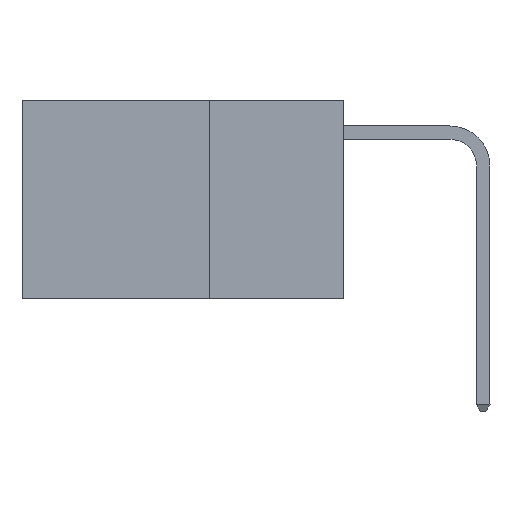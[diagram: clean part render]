
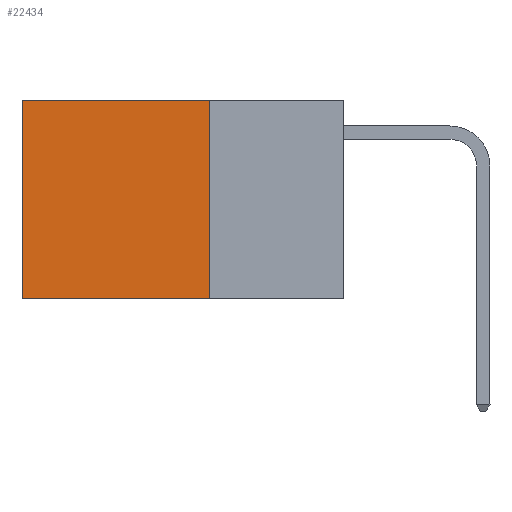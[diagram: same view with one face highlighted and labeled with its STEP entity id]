
A CAD part, left-side view. The second image highlights one B-rep face of the part: STEP entity #22434.
In plain terms, the highlighted planar face has unit normal (-1, 0, 0).
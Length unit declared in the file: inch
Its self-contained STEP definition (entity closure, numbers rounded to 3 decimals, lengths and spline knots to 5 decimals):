
#452 = VERTEX_POINT ( 'NONE', #15497 ) ;
#905 = DIRECTION ( 'NONE',  ( 0., 0., -1. ) ) ;
#1413 = ORIENTED_EDGE ( 'NONE', *, *, #18314, .T. ) ;
#1523 = ORIENTED_EDGE ( 'NONE', *, *, #17590, .F. ) ;
#2124 = AXIS2_PLACEMENT_3D ( 'NONE', #5800, #19646, #9467 ) ;
#4443 = FACE_OUTER_BOUND ( 'NONE', #20118, .T. ) ;
#4970 = VECTOR ( 'NONE', #7702, 39.37008 ) ;
#5228 = DIRECTION ( 'NONE',  ( 0., 1., 0. ) ) ;
#5557 = LINE ( 'NONE', #19661, #4970 ) ;
#5603 = CARTESIAN_POINT ( 'NONE',  ( 0.2625, 0.25, 0. ) ) ;
#5800 = CARTESIAN_POINT ( 'NONE',  ( 0.2625, 0.25, 0. ) ) ;
#7702 = DIRECTION ( 'NONE',  ( 0., 0., -1. ) ) ;
#8188 = VECTOR ( 'NONE', #9910, 39.37008 ) ;
#8768 = VERTEX_POINT ( 'NONE', #12244 ) ;
#9467 = DIRECTION ( 'NONE',  ( 0., 0., -1. ) ) ;
#9661 = CARTESIAN_POINT ( 'NONE',  ( 0.2625, 0.6, 0. ) ) ;
#9910 = DIRECTION ( 'NONE',  ( 0., 1., 0. ) ) ;
#10698 = EDGE_CURVE ( 'NONE', #452, #15655, #19835, .T. ) ;
#11452 = VECTOR ( 'NONE', #5228, 39.37008 ) ;
#12244 = CARTESIAN_POINT ( 'NONE',  ( 0.2625, 0.25, -0.37 ) ) ;
#12859 = LINE ( 'NONE', #21720, #8188 ) ;
#13595 = LINE ( 'NONE', #15285, #21959 ) ;
#14834 = CARTESIAN_POINT ( 'NONE',  ( 0.2625, 0.6, -0.37 ) ) ;
#15219 = EDGE_CURVE ( 'NONE', #8768, #18791, #12859, .T. ) ;
#15285 = CARTESIAN_POINT ( 'NONE',  ( 0.2625, 0.6, 0. ) ) ;
#15357 = ORIENTED_EDGE ( 'NONE', *, *, #15219, .F. ) ;
#15497 = CARTESIAN_POINT ( 'NONE',  ( 0.2625, 0.25, 0. ) ) ;
#15655 = VERTEX_POINT ( 'NONE', #9661 ) ;
#17590 = EDGE_CURVE ( 'NONE', #452, #8768, #5557, .T. ) ;
#17978 = PLANE ( 'NONE',  #2124 ) ;
#18314 = EDGE_CURVE ( 'NONE', #15655, #18791, #13595, .T. ) ;
#18791 = VERTEX_POINT ( 'NONE', #14834 ) ;
#19646 = DIRECTION ( 'NONE',  ( 1., 0., 0. ) ) ;
#19661 = CARTESIAN_POINT ( 'NONE',  ( 0.2625, 0.25, 0. ) ) ;
#19835 = LINE ( 'NONE', #5603, #11452 ) ;
#20118 = EDGE_LOOP ( 'NONE', ( #1413, #15357, #1523, #22451 ) ) ;
#21720 = CARTESIAN_POINT ( 'NONE',  ( 0.2625, 0.25, -0.37 ) ) ;
#21959 = VECTOR ( 'NONE', #905, 39.37008 ) ;
#22434 = ADVANCED_FACE ( 'NONE', ( #4443 ), #17978, .F. ) ;
#22451 = ORIENTED_EDGE ( 'NONE', *, *, #10698, .T. ) ;
